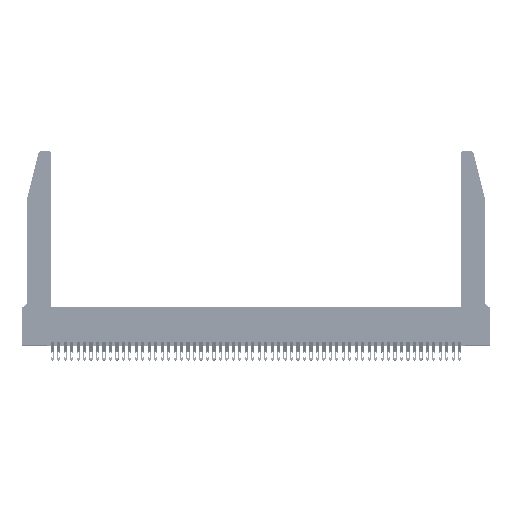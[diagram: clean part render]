
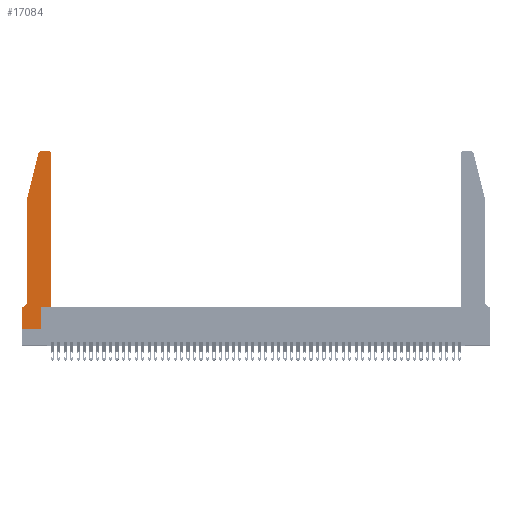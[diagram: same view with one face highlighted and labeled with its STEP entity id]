
A CAD part, top view. The second image highlights one B-rep face of the part: STEP entity #17084.
In plain terms, the highlighted planar face has unit normal (0, 0, 1).
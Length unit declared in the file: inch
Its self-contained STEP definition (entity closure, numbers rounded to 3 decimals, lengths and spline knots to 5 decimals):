
#1611 = VERTEX_POINT ( 'NONE', #45846 ) ;
#2856 = CARTESIAN_POINT ( 'NONE',  ( 0.4505, 0.35, 0.37 ) ) ;
#3760 = CARTESIAN_POINT ( 'NONE',  ( 0.284, 2.72, 0.37 ) ) ;
#4116 = DIRECTION ( 'NONE',  ( 0., 0., 1. ) ) ;
#4305 = CARTESIAN_POINT ( 'NONE',  ( 0.2605, 2.75, 0.37 ) ) ;
#4559 = CARTESIAN_POINT ( 'NONE',  ( 0.2865, 0.35, 0.37 ) ) ;
#4715 = ORIENTED_EDGE ( 'NONE', *, *, #21417, .T. ) ;
#5212 = DIRECTION ( 'NONE',  ( -0.239, -0.971, 0. ) ) ;
#5669 = EDGE_CURVE ( 'NONE', #6753, #8586, #24663, .T. ) ;
#5851 = EDGE_CURVE ( 'NONE', #10971, #37607, #28227, .T. ) ;
#6750 = ORIENTED_EDGE ( 'NONE', *, *, #25923, .T. ) ;
#6753 = VERTEX_POINT ( 'NONE', #48438 ) ;
#7187 = VECTOR ( 'NONE', #18605, 39.37008 ) ;
#7791 = VERTEX_POINT ( 'NONE', #26396 ) ;
#8091 = EDGE_CURVE ( 'NONE', #36282, #16673, #43789, .T. ) ;
#8586 = VERTEX_POINT ( 'NONE', #23485 ) ;
#8636 = CIRCLE ( 'NONE', #32991, 0.07 ) ;
#8673 = VECTOR ( 'NONE', #25015, 39.37008 ) ;
#8725 = CARTESIAN_POINT ( 'NONE',  ( 0.0055, 0.42, 0.37 ) ) ;
#8784 = DIRECTION ( 'NONE',  ( 1., 0., 0. ) ) ;
#9540 = LINE ( 'NONE', #41537, #17132 ) ;
#9759 = AXIS2_PLACEMENT_3D ( 'NONE', #3760, #4116, #36441 ) ;
#10971 = VERTEX_POINT ( 'NONE', #31273 ) ;
#11161 = VERTEX_POINT ( 'NONE', #31813 ) ;
#12199 = CARTESIAN_POINT ( 'NONE',  ( 0.0755, 2., 0.37 ) ) ;
#12509 = VECTOR ( 'NONE', #20585, 39.37008 ) ;
#12647 = CARTESIAN_POINT ( 'NONE',  ( 0.0055, 0.35, 0.37 ) ) ;
#12708 = DIRECTION ( 'NONE',  ( 0., 0., 1. ) ) ;
#13771 = LINE ( 'NONE', #40561, #12509 ) ;
#13780 = DIRECTION ( 'NONE',  ( 0., 1., 0. ) ) ;
#15013 = CARTESIAN_POINT ( 'NONE',  ( 0.4205, 2.75, 0.37 ) ) ;
#16673 = VERTEX_POINT ( 'NONE', #34394 ) ;
#17084 = ADVANCED_FACE ( 'NONE', ( #47291 ), #17430, .T. ) ;
#17132 = VECTOR ( 'NONE', #17369, 39.37008 ) ;
#17369 = DIRECTION ( 'NONE',  ( -1., 0., 0. ) ) ;
#17430 = PLANE ( 'NONE',  #25386 ) ;
#17609 = CIRCLE ( 'NONE', #9759, 0.03 ) ;
#17739 = CARTESIAN_POINT ( 'NONE',  ( 0.0755, 2., 0.37 ) ) ;
#18114 = CARTESIAN_POINT ( 'NONE',  ( 0.4205, 2.72, 0.37 ) ) ;
#18155 = CARTESIAN_POINT ( 'NONE',  ( 0.4505, 0.35, 0.37 ) ) ;
#18605 = DIRECTION ( 'NONE',  ( 1., 0., 0. ) ) ;
#18751 = VECTOR ( 'NONE', #13780, 39.37008 ) ;
#19869 = LINE ( 'NONE', #17739, #35706 ) ;
#20255 = EDGE_CURVE ( 'NONE', #11161, #6753, #19869, .T. ) ;
#20585 = DIRECTION ( 'NONE',  ( 1., 0., 0. ) ) ;
#21200 = DIRECTION ( 'NONE',  ( -1., 0., 0. ) ) ;
#21417 = EDGE_CURVE ( 'NONE', #7791, #26669, #32460, .T. ) ;
#21560 = CARTESIAN_POINT ( 'NONE',  ( 0., 0., 0.37 ) ) ;
#22279 = VECTOR ( 'NONE', #48312, 39.37008 ) ;
#22693 = ORIENTED_EDGE ( 'NONE', *, *, #8091, .T. ) ;
#23485 = CARTESIAN_POINT ( 'NONE',  ( 0.0755, 0.42, 0.37 ) ) ;
#24663 = LINE ( 'NONE', #12199, #46874 ) ;
#25015 = DIRECTION ( 'NONE',  ( 0., 1., 0. ) ) ;
#25275 = CIRCLE ( 'NONE', #49192, 0.03 ) ;
#25386 = AXIS2_PLACEMENT_3D ( 'NONE', #41077, #12708, #8784 ) ;
#25850 = EDGE_CURVE ( 'NONE', #26669, #36270, #13771, .T. ) ;
#25923 = EDGE_CURVE ( 'NONE', #36270, #1611, #35813, .T. ) ;
#26396 = CARTESIAN_POINT ( 'NONE',  ( 0., 0.35, 0.37 ) ) ;
#26652 = CARTESIAN_POINT ( 'NONE',  ( 0.2865, 0., 0.37 ) ) ;
#26669 = VERTEX_POINT ( 'NONE', #21560 ) ;
#28227 = LINE ( 'NONE', #18155, #18751 ) ;
#29189 = DIRECTION ( 'NONE',  ( 0., 0., -1. ) ) ;
#29544 = EDGE_CURVE ( 'NONE', #37607, #36282, #25275, .T. ) ;
#31273 = CARTESIAN_POINT ( 'NONE',  ( 0.4505, 0.35, 0.37 ) ) ;
#31813 = CARTESIAN_POINT ( 'NONE',  ( 0.25487, 2.72718, 0.37 ) ) ;
#31879 = ORIENTED_EDGE ( 'NONE', *, *, #25850, .T. ) ;
#32460 = LINE ( 'NONE', #49186, #44506 ) ;
#32991 = AXIS2_PLACEMENT_3D ( 'NONE', #8725, #29189, #21200 ) ;
#34257 = CARTESIAN_POINT ( 'NONE',  ( 0.4505, 2.72, 0.37 ) ) ;
#34394 = CARTESIAN_POINT ( 'NONE',  ( 0.284, 2.75, 0.37 ) ) ;
#34578 = EDGE_LOOP ( 'NONE', ( #22693, #37886, #40967, #49538, #42552, #45526, #4715, #31879, #6750, #49412, #46736, #51728 ) ) ;
#35706 = VECTOR ( 'NONE', #5212, 39.37008 ) ;
#35813 = LINE ( 'NONE', #4559, #8673 ) ;
#36270 = VERTEX_POINT ( 'NONE', #26652 ) ;
#36282 = VERTEX_POINT ( 'NONE', #15013 ) ;
#36441 = DIRECTION ( 'NONE',  ( 1., 0., 0. ) ) ;
#37607 = VERTEX_POINT ( 'NONE', #34257 ) ;
#37886 = ORIENTED_EDGE ( 'NONE', *, *, #51906, .T. ) ;
#37895 = DIRECTION ( 'NONE',  ( 0., 0., 1. ) ) ;
#40406 = DIRECTION ( 'NONE',  ( 0., -1., 0. ) ) ;
#40561 = CARTESIAN_POINT ( 'NONE',  ( 0., 0., 0.37 ) ) ;
#40967 = ORIENTED_EDGE ( 'NONE', *, *, #20255, .T. ) ;
#41077 = CARTESIAN_POINT ( 'NONE',  ( 0., 0.35, 0.37 ) ) ;
#41537 = CARTESIAN_POINT ( 'NONE',  ( 0.0755, 0.35, 0.37 ) ) ;
#42552 = ORIENTED_EDGE ( 'NONE', *, *, #50129, .T. ) ;
#43710 = EDGE_CURVE ( 'NONE', #49987, #7791, #9540, .T. ) ;
#43789 = LINE ( 'NONE', #4305, #22279 ) ;
#44506 = VECTOR ( 'NONE', #45283, 39.37008 ) ;
#45283 = DIRECTION ( 'NONE',  ( 0., -1., 0. ) ) ;
#45326 = EDGE_CURVE ( 'NONE', #1611, #10971, #47650, .T. ) ;
#45526 = ORIENTED_EDGE ( 'NONE', *, *, #43710, .T. ) ;
#45846 = CARTESIAN_POINT ( 'NONE',  ( 0.2865, 0.35, 0.37 ) ) ;
#46053 = DIRECTION ( 'NONE',  ( 1., 0., 0. ) ) ;
#46736 = ORIENTED_EDGE ( 'NONE', *, *, #5851, .T. ) ;
#46874 = VECTOR ( 'NONE', #40406, 39.37008 ) ;
#47291 = FACE_OUTER_BOUND ( 'NONE', #34578, .T. ) ;
#47650 = LINE ( 'NONE', #2856, #7187 ) ;
#48312 = DIRECTION ( 'NONE',  ( -1., 0., 0. ) ) ;
#48438 = CARTESIAN_POINT ( 'NONE',  ( 0.0755, 2., 0.37 ) ) ;
#49186 = CARTESIAN_POINT ( 'NONE',  ( 0., 0., 0.37 ) ) ;
#49192 = AXIS2_PLACEMENT_3D ( 'NONE', #18114, #37895, #46053 ) ;
#49412 = ORIENTED_EDGE ( 'NONE', *, *, #45326, .T. ) ;
#49538 = ORIENTED_EDGE ( 'NONE', *, *, #5669, .T. ) ;
#49987 = VERTEX_POINT ( 'NONE', #12647 ) ;
#50129 = EDGE_CURVE ( 'NONE', #8586, #49987, #8636, .T. ) ;
#51728 = ORIENTED_EDGE ( 'NONE', *, *, #29544, .T. ) ;
#51906 = EDGE_CURVE ( 'NONE', #16673, #11161, #17609, .T. ) ;
